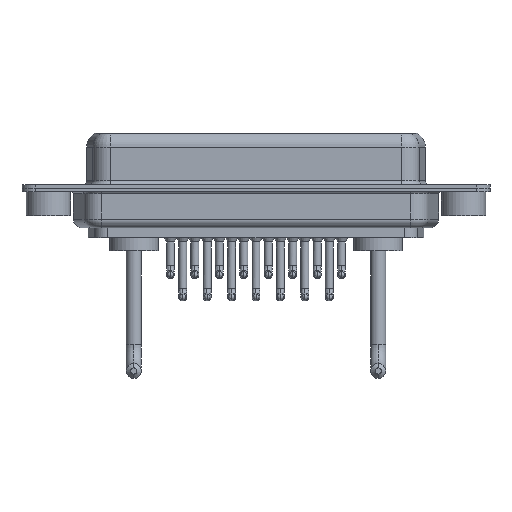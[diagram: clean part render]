
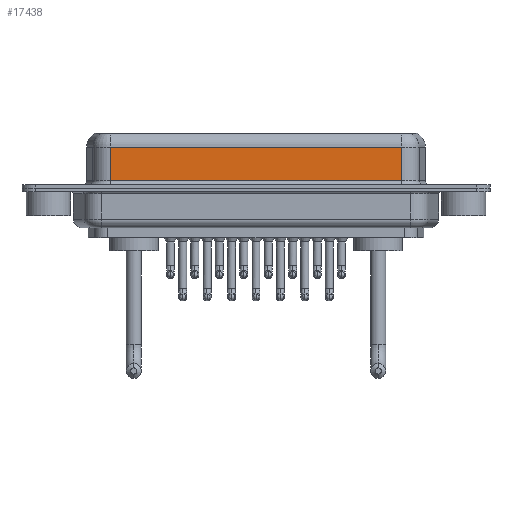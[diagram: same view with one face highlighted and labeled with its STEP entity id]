
A CAD part, front view. The second image highlights one B-rep face of the part: STEP entity #17438.
In plain terms, the highlighted planar face has unit normal (0, -1, 0).
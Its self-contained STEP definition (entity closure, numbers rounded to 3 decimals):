
#1534 = LINE ( 'NONE', #7968, #7767 ) ;
#1657 = AXIS2_PLACEMENT_3D ( 'NONE', #7731, #14570, #10884 ) ;
#1698 = DIRECTION ( 'NONE',  ( -1., 0., 0. ) ) ;
#2486 = LINE ( 'NONE', #18582, #5182 ) ;
#3420 = DIRECTION ( 'NONE',  ( 1., 0., 0. ) ) ;
#4749 = CARTESIAN_POINT ( 'NONE',  ( 7.013, -3.95, 0.9 ) ) ;
#5182 = VECTOR ( 'NONE', #7225, 1000. ) ;
#5270 = CARTESIAN_POINT ( 'NONE',  ( 7.013, -3.95, 4.65 ) ) ;
#6238 = FACE_OUTER_BOUND ( 'NONE', #10395, .T. ) ;
#6759 = EDGE_CURVE ( 'NONE', #8901, #12829, #1534, .T. ) ;
#7225 = DIRECTION ( 'NONE',  ( 0., 0., -1. ) ) ;
#7731 = CARTESIAN_POINT ( 'NONE',  ( 40.037, -3.95, 6.4 ) ) ;
#7767 = VECTOR ( 'NONE', #3420, 1000. ) ;
#7968 = CARTESIAN_POINT ( 'NONE',  ( 40.037, -3.95, 0.9 ) ) ;
#8114 = ORIENTED_EDGE ( 'NONE', *, *, #10888, .F. ) ;
#8901 = VERTEX_POINT ( 'NONE', #4749 ) ;
#9297 = ORIENTED_EDGE ( 'NONE', *, *, #10657, .T. ) ;
#10395 = EDGE_LOOP ( 'NONE', ( #8114, #9297, #20058, #15568 ) ) ;
#10657 = EDGE_CURVE ( 'NONE', #12527, #14029, #17911, .T. ) ;
#10884 = DIRECTION ( 'NONE',  ( 0., 0., 1. ) ) ;
#10888 = EDGE_CURVE ( 'NONE', #12527, #12829, #18015, .T. ) ;
#11807 = EDGE_CURVE ( 'NONE', #14029, #8901, #2486, .T. ) ;
#12527 = VERTEX_POINT ( 'NONE', #19974 ) ;
#12829 = VERTEX_POINT ( 'NONE', #16188 ) ;
#13493 = CARTESIAN_POINT ( 'NONE',  ( 40.037, -3.95, 6.4 ) ) ;
#14029 = VERTEX_POINT ( 'NONE', #5270 ) ;
#14570 = DIRECTION ( 'NONE',  ( 0., 1., 0. ) ) ;
#14608 = VECTOR ( 'NONE', #1698, 1000. ) ;
#15568 = ORIENTED_EDGE ( 'NONE', *, *, #6759, .T. ) ;
#16127 = CARTESIAN_POINT ( 'NONE',  ( 40.037, -3.95, 4.65 ) ) ;
#16188 = CARTESIAN_POINT ( 'NONE',  ( 40.037, -3.95, 0.9 ) ) ;
#16543 = VECTOR ( 'NONE', #19893, 1000. ) ;
#17438 = ADVANCED_FACE ( 'NONE', ( #6238 ), #20644, .F. ) ;
#17911 = LINE ( 'NONE', #16127, #14608 ) ;
#18015 = LINE ( 'NONE', #13493, #16543 ) ;
#18582 = CARTESIAN_POINT ( 'NONE',  ( 7.013, -3.95, 6.4 ) ) ;
#19893 = DIRECTION ( 'NONE',  ( 0., 0., -1. ) ) ;
#19974 = CARTESIAN_POINT ( 'NONE',  ( 40.037, -3.95, 4.65 ) ) ;
#20058 = ORIENTED_EDGE ( 'NONE', *, *, #11807, .T. ) ;
#20644 = PLANE ( 'NONE',  #1657 ) ;
